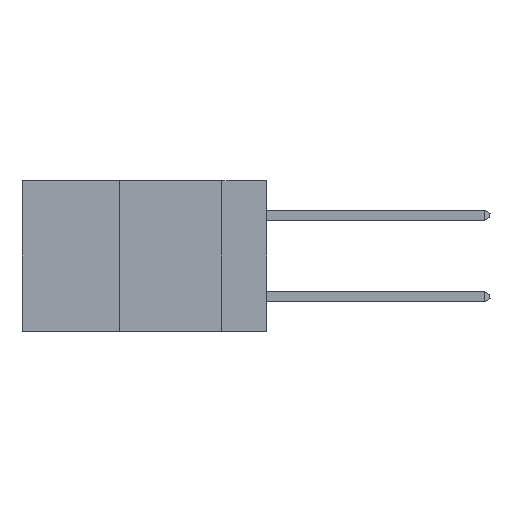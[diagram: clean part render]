
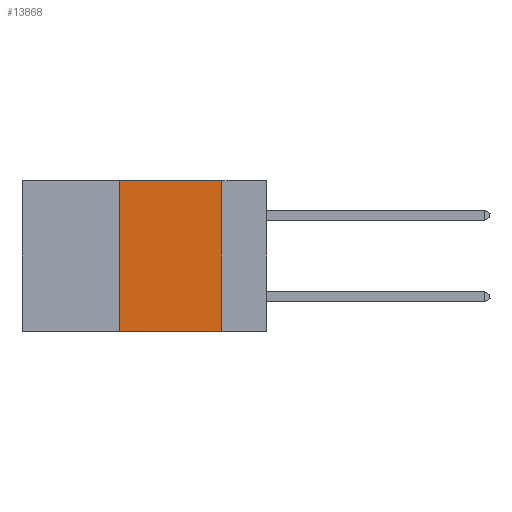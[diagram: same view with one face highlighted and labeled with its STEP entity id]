
A CAD part, left-side view. The second image highlights one B-rep face of the part: STEP entity #13868.
In plain terms, the highlighted planar face has unit normal (-1, 0, 0).
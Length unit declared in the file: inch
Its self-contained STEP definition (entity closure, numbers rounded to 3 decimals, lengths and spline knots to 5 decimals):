
#156 = ORIENTED_EDGE ( 'NONE', *, *, #4815, .T. ) ;
#684 = AXIS2_PLACEMENT_3D ( 'NONE', #6685, #16316, #12642 ) ;
#2022 = CARTESIAN_POINT ( 'NONE',  ( 0., 0.11, 0. ) ) ;
#3522 = VECTOR ( 'NONE', #17424, 39.37008 ) ;
#4624 = VECTOR ( 'NONE', #24030, 39.37008 ) ;
#4759 = VECTOR ( 'NONE', #24588, 39.37008 ) ;
#4815 = EDGE_CURVE ( 'NONE', #24606, #6020, #23686, .T. ) ;
#6020 = VERTEX_POINT ( 'NONE', #23764 ) ;
#6685 = CARTESIAN_POINT ( 'NONE',  ( 0., 0.6, 0. ) ) ;
#7941 = EDGE_CURVE ( 'NONE', #24606, #12752, #22873, .T. ) ;
#9638 = ORIENTED_EDGE ( 'NONE', *, *, #7941, .F. ) ;
#9686 = CARTESIAN_POINT ( 'NONE',  ( 0., 0.36, 0. ) ) ;
#10201 = LINE ( 'NONE', #10350, #4759 ) ;
#10350 = CARTESIAN_POINT ( 'NONE',  ( 0., 0.6, 0. ) ) ;
#10594 = CARTESIAN_POINT ( 'NONE',  ( 0., 0.11, 0. ) ) ;
#12060 = EDGE_CURVE ( 'NONE', #12752, #12370, #10201, .T. ) ;
#12370 = VERTEX_POINT ( 'NONE', #2022 ) ;
#12384 = FACE_OUTER_BOUND ( 'NONE', #13394, .T. ) ;
#12642 = DIRECTION ( 'NONE',  ( 0., 0., -1. ) ) ;
#12731 = PLANE ( 'NONE',  #684 ) ;
#12752 = VERTEX_POINT ( 'NONE', #16233 ) ;
#13394 = EDGE_LOOP ( 'NONE', ( #26073, #26294, #9638, #156 ) ) ;
#13868 = ADVANCED_FACE ( 'NONE', ( #12384 ), #12731, .F. ) ;
#15410 = EDGE_CURVE ( 'NONE', #12370, #6020, #23630, .T. ) ;
#16233 = CARTESIAN_POINT ( 'NONE',  ( 0., 0.36, 0. ) ) ;
#16316 = DIRECTION ( 'NONE',  ( 1., 0., 0. ) ) ;
#17424 = DIRECTION ( 'NONE',  ( 0., -1., 0. ) ) ;
#18054 = CARTESIAN_POINT ( 'NONE',  ( 0., 0.36, -0.37 ) ) ;
#21378 = CARTESIAN_POINT ( 'NONE',  ( 0., 0.6, -0.37 ) ) ;
#21397 = VECTOR ( 'NONE', #24914, 39.37008 ) ;
#22873 = LINE ( 'NONE', #9686, #4624 ) ;
#23630 = LINE ( 'NONE', #10594, #21397 ) ;
#23686 = LINE ( 'NONE', #21378, #3522 ) ;
#23764 = CARTESIAN_POINT ( 'NONE',  ( 0., 0.11, -0.37 ) ) ;
#24030 = DIRECTION ( 'NONE',  ( 0., 0., 1. ) ) ;
#24588 = DIRECTION ( 'NONE',  ( 0., -1., 0. ) ) ;
#24606 = VERTEX_POINT ( 'NONE', #18054 ) ;
#24914 = DIRECTION ( 'NONE',  ( 0., 0., -1. ) ) ;
#26073 = ORIENTED_EDGE ( 'NONE', *, *, #15410, .F. ) ;
#26294 = ORIENTED_EDGE ( 'NONE', *, *, #12060, .F. ) ;
